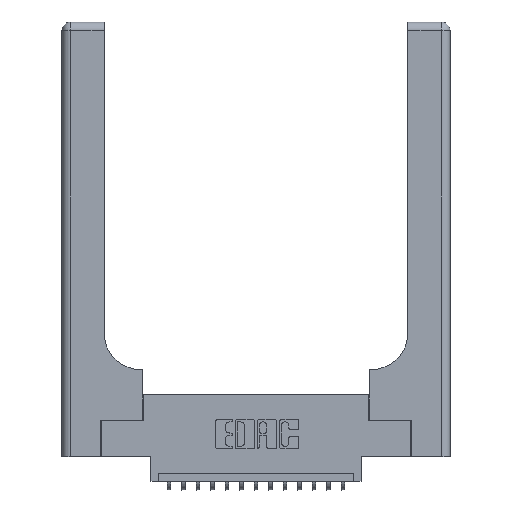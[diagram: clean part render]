
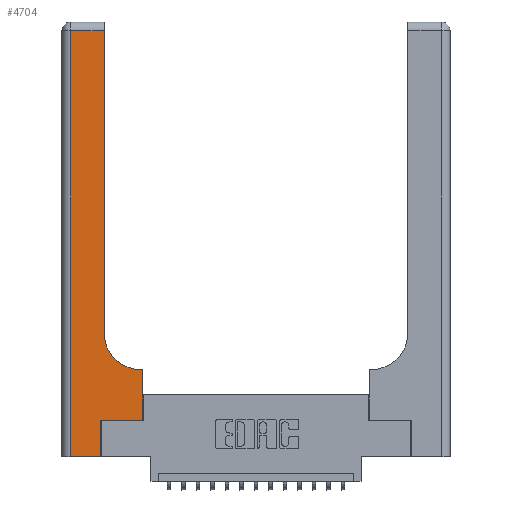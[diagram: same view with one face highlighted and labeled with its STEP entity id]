
A CAD part, top view. The second image highlights one B-rep face of the part: STEP entity #4704.
In plain terms, the highlighted planar face has unit normal (0, 0, 1).
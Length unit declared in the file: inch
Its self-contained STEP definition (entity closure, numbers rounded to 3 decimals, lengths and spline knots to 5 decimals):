
#293 = CARTESIAN_POINT ( 'NONE',  ( 0.2915, 3., 0.37 ) ) ;
#605 = CARTESIAN_POINT ( 'NONE',  ( 0.5415, 0.6, 0.37 ) ) ;
#616 = CARTESIAN_POINT ( 'NONE',  ( 0.2915, 2.94, 0.37 ) ) ;
#845 = DIRECTION ( 'NONE',  ( 0., -1., 0. ) ) ;
#1261 = VECTOR ( 'NONE', #17598, 39.37008 ) ;
#1340 = CARTESIAN_POINT ( 'NONE',  ( 0.269, 0., 0.37 ) ) ;
#2204 = ORIENTED_EDGE ( 'NONE', *, *, #14682, .T. ) ;
#2476 = VERTEX_POINT ( 'NONE', #1340 ) ;
#2487 = VERTEX_POINT ( 'NONE', #17597 ) ;
#2546 = LINE ( 'NONE', #8468, #18666 ) ;
#3233 = LINE ( 'NONE', #13869, #4610 ) ;
#3719 = EDGE_CURVE ( 'NONE', #18501, #14759, #16036, .T. ) ;
#4307 = DIRECTION ( 'NONE',  ( 1., 0., 0. ) ) ;
#4610 = VECTOR ( 'NONE', #7971, 39.37008 ) ;
#4704 = ADVANCED_FACE ( 'NONE', ( #12599 ), #6754, .F. ) ;
#4967 = VECTOR ( 'NONE', #15344, 39.37008 ) ;
#5209 = ORIENTED_EDGE ( 'NONE', *, *, #17021, .T. ) ;
#5835 = CARTESIAN_POINT ( 'NONE',  ( 0.5585, 0.6, 0.37 ) ) ;
#5855 = VERTEX_POINT ( 'NONE', #5835 ) ;
#6070 = DIRECTION ( 'NONE',  ( 0., 0., -1. ) ) ;
#6181 = DIRECTION ( 'NONE',  ( 0., 1., 0. ) ) ;
#6727 = ORIENTED_EDGE ( 'NONE', *, *, #16914, .T. ) ;
#6754 = PLANE ( 'NONE',  #12017 ) ;
#6886 = DIRECTION ( 'NONE',  ( 0., 0., -1. ) ) ;
#6943 = ORIENTED_EDGE ( 'NONE', *, *, #11101, .T. ) ;
#7286 = VECTOR ( 'NONE', #19102, 39.37008 ) ;
#7531 = CARTESIAN_POINT ( 'NONE',  ( 0.2915, 0.6, 0.37 ) ) ;
#7815 = AXIS2_PLACEMENT_3D ( 'NONE', #9785, #6070, #15239 ) ;
#7925 = VERTEX_POINT ( 'NONE', #605 ) ;
#7971 = DIRECTION ( 'NONE',  ( 0., 1., 0. ) ) ;
#8368 = DIRECTION ( 'NONE',  ( -1., 0., 0. ) ) ;
#8468 = CARTESIAN_POINT ( 'NONE',  ( 0.06, 3., 0.37 ) ) ;
#8602 = CARTESIAN_POINT ( 'NONE',  ( 0.269, 0.25, 0.37 ) ) ;
#8691 = CARTESIAN_POINT ( 'NONE',  ( 0., 0., 0.37 ) ) ;
#9111 = ORIENTED_EDGE ( 'NONE', *, *, #3719, .T. ) ;
#9161 = CIRCLE ( 'NONE', #7815, 0.25 ) ;
#9176 = EDGE_CURVE ( 'NONE', #7925, #9297, #9161, .T. ) ;
#9297 = VERTEX_POINT ( 'NONE', #14647 ) ;
#9491 = CARTESIAN_POINT ( 'NONE',  ( 0.5585, 0.25, 0.37 ) ) ;
#9785 = CARTESIAN_POINT ( 'NONE',  ( 0.5415, 0.85, 0.37 ) ) ;
#10009 = LINE ( 'NONE', #293, #14391 ) ;
#10463 = VECTOR ( 'NONE', #14845, 39.37008 ) ;
#11101 = EDGE_CURVE ( 'NONE', #9297, #18501, #10009, .T. ) ;
#11183 = CARTESIAN_POINT ( 'NONE',  ( 0., 3., 0.37 ) ) ;
#11361 = EDGE_LOOP ( 'NONE', ( #6943, #9111, #5209, #2204, #6727, #15707, #13331, #14882, #16277 ) ) ;
#12017 = AXIS2_PLACEMENT_3D ( 'NONE', #11183, #6886, #8368 ) ;
#12599 = FACE_OUTER_BOUND ( 'NONE', #11361, .T. ) ;
#12691 = EDGE_CURVE ( 'NONE', #2487, #5855, #18117, .T. ) ;
#13331 = ORIENTED_EDGE ( 'NONE', *, *, #12691, .T. ) ;
#13869 = CARTESIAN_POINT ( 'NONE',  ( 0.269, 0., 0.37 ) ) ;
#14177 = LINE ( 'NONE', #8691, #1261 ) ;
#14375 = LINE ( 'NONE', #7531, #10463 ) ;
#14391 = VECTOR ( 'NONE', #6181, 39.37008 ) ;
#14647 = CARTESIAN_POINT ( 'NONE',  ( 0.2915, 0.85, 0.37 ) ) ;
#14682 = EDGE_CURVE ( 'NONE', #17524, #2476, #14177, .T. ) ;
#14759 = VERTEX_POINT ( 'NONE', #17352 ) ;
#14845 = DIRECTION ( 'NONE',  ( -1., 0., 0. ) ) ;
#14877 = EDGE_CURVE ( 'NONE', #5855, #7925, #14375, .T. ) ;
#14882 = ORIENTED_EDGE ( 'NONE', *, *, #14877, .T. ) ;
#15239 = DIRECTION ( 'NONE',  ( 1., 0., 0. ) ) ;
#15344 = DIRECTION ( 'NONE',  ( 0., 1., 0. ) ) ;
#15707 = ORIENTED_EDGE ( 'NONE', *, *, #17036, .T. ) ;
#16036 = LINE ( 'NONE', #17734, #7286 ) ;
#16277 = ORIENTED_EDGE ( 'NONE', *, *, #9176, .T. ) ;
#16914 = EDGE_CURVE ( 'NONE', #2476, #18178, #3233, .T. ) ;
#17021 = EDGE_CURVE ( 'NONE', #14759, #17524, #2546, .T. ) ;
#17036 = EDGE_CURVE ( 'NONE', #18178, #2487, #18889, .T. ) ;
#17352 = CARTESIAN_POINT ( 'NONE',  ( 0.06, 2.94, 0.37 ) ) ;
#17524 = VERTEX_POINT ( 'NONE', #18520 ) ;
#17597 = CARTESIAN_POINT ( 'NONE',  ( 0.5585, 0.25, 0.37 ) ) ;
#17598 = DIRECTION ( 'NONE',  ( 1., 0., 0. ) ) ;
#17734 = CARTESIAN_POINT ( 'NONE',  ( 0., 2.94, 0.37 ) ) ;
#18117 = LINE ( 'NONE', #9491, #4967 ) ;
#18178 = VERTEX_POINT ( 'NONE', #8602 ) ;
#18431 = VECTOR ( 'NONE', #4307, 39.37008 ) ;
#18501 = VERTEX_POINT ( 'NONE', #616 ) ;
#18520 = CARTESIAN_POINT ( 'NONE',  ( 0.06, 0., 0.37 ) ) ;
#18666 = VECTOR ( 'NONE', #845, 39.37008 ) ;
#18889 = LINE ( 'NONE', #18928, #18431 ) ;
#18928 = CARTESIAN_POINT ( 'NONE',  ( 0.269, 0.25, 0.37 ) ) ;
#19102 = DIRECTION ( 'NONE',  ( -1., 0., 0. ) ) ;
